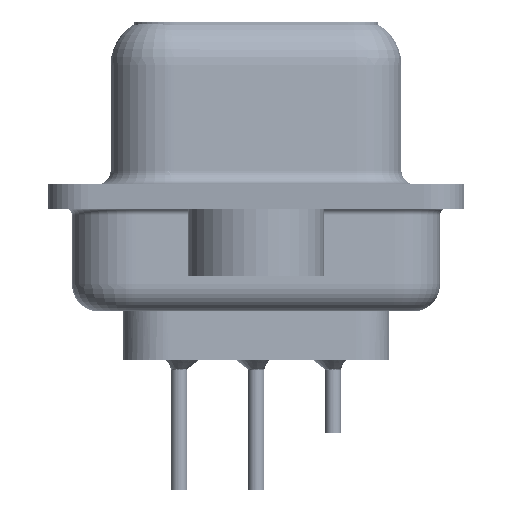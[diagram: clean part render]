
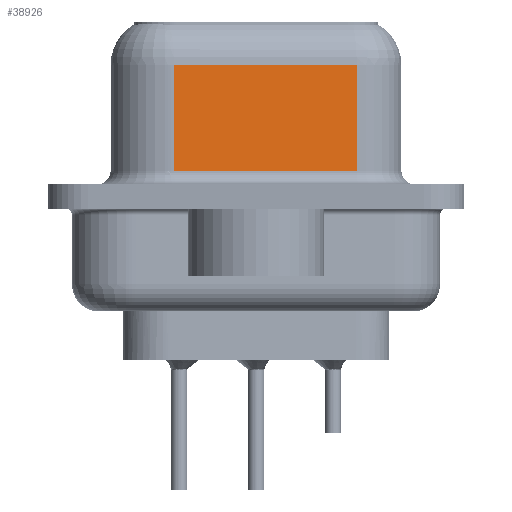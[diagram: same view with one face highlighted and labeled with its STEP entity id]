
A CAD part, left-side view. The second image highlights one B-rep face of the part: STEP entity #38926.
In plain terms, the highlighted planar face has unit normal (-0.985, -0.174, 0).
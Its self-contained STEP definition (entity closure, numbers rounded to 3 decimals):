
#381 = VERTEX_POINT ( 'NONE', #27605 ) ;
#1342 = ORIENTED_EDGE ( 'NONE', *, *, #34248, .T. ) ;
#1644 = VECTOR ( 'NONE', #3323, 1000. ) ;
#2850 = EDGE_LOOP ( 'NONE', ( #27275, #1342, #25609, #38008 ) ) ;
#2908 = VERTEX_POINT ( 'NONE', #32846 ) ;
#3136 = DIRECTION ( 'NONE',  ( 0.985, 0.174, 0. ) ) ;
#3323 = DIRECTION ( 'NONE',  ( 0., 0., -1. ) ) ;
#7084 = LINE ( 'NONE', #20134, #37037 ) ;
#7764 = VERTEX_POINT ( 'NONE', #40355 ) ;
#10177 = LINE ( 'NONE', #22818, #1644 ) ;
#10393 = VERTEX_POINT ( 'NONE', #26234 ) ;
#11942 = AXIS2_PLACEMENT_3D ( 'NONE', #36114, #3136, #26240 ) ;
#12048 = VECTOR ( 'NONE', #26095, 1000. ) ;
#12418 = LINE ( 'NONE', #38353, #12048 ) ;
#12934 = DIRECTION ( 'NONE',  ( 0., 0., -1. ) ) ;
#17749 = EDGE_CURVE ( 'NONE', #7764, #381, #10177, .T. ) ;
#20134 = CARTESIAN_POINT ( 'NONE',  ( 5.621, -3.722, 4.85 ) ) ;
#20286 = EDGE_CURVE ( 'NONE', #10393, #2908, #42267, .T. ) ;
#22149 = EDGE_CURVE ( 'NONE', #2908, #381, #12418, .T. ) ;
#22427 = PLANE ( 'NONE',  #11942 ) ;
#22818 = CARTESIAN_POINT ( 'NONE',  ( 5.621, -3.722, 6.6 ) ) ;
#22843 = FACE_OUTER_BOUND ( 'NONE', #2850, .T. ) ;
#24282 = VECTOR ( 'NONE', #12934, 1000. ) ;
#25609 = ORIENTED_EDGE ( 'NONE', *, *, #20286, .T. ) ;
#26095 = DIRECTION ( 'NONE',  ( 0.174, -0.985, 0. ) ) ;
#26234 = CARTESIAN_POINT ( 'NONE',  ( 4.43, 3.028, 4.85 ) ) ;
#26240 = DIRECTION ( 'NONE',  ( -0.174, 0.985, 0. ) ) ;
#27275 = ORIENTED_EDGE ( 'NONE', *, *, #17749, .F. ) ;
#27605 = CARTESIAN_POINT ( 'NONE',  ( 5.621, -3.722, 0.95 ) ) ;
#29166 = CARTESIAN_POINT ( 'NONE',  ( 4.43, 3.028, 6.6 ) ) ;
#32846 = CARTESIAN_POINT ( 'NONE',  ( 4.43, 3.028, 0.95 ) ) ;
#33176 = DIRECTION ( 'NONE',  ( -0.174, 0.985, 0. ) ) ;
#34248 = EDGE_CURVE ( 'NONE', #7764, #10393, #7084, .T. ) ;
#36114 = CARTESIAN_POINT ( 'NONE',  ( 5.621, -3.722, 6.6 ) ) ;
#37037 = VECTOR ( 'NONE', #33176, 1000. ) ;
#38008 = ORIENTED_EDGE ( 'NONE', *, *, #22149, .T. ) ;
#38353 = CARTESIAN_POINT ( 'NONE',  ( 5.621, -3.722, 0.95 ) ) ;
#38926 = ADVANCED_FACE ( 'NONE', ( #22843 ), #22427, .F. ) ;
#40355 = CARTESIAN_POINT ( 'NONE',  ( 5.621, -3.722, 4.85 ) ) ;
#42267 = LINE ( 'NONE', #29166, #24282 ) ;
